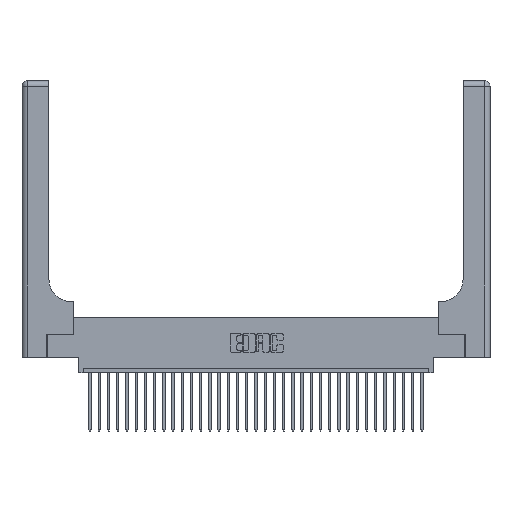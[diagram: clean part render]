
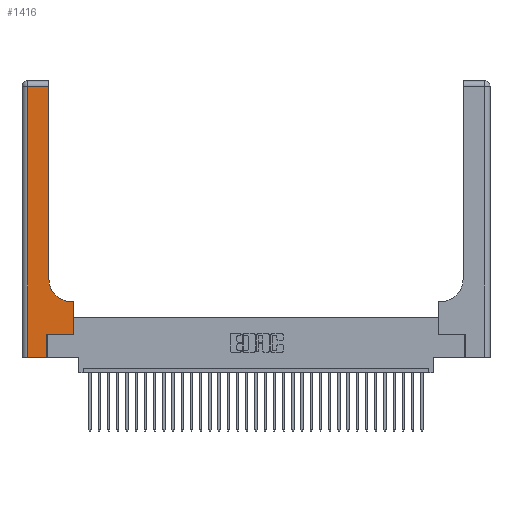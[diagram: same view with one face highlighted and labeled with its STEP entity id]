
A CAD part, top view. The second image highlights one B-rep face of the part: STEP entity #1416.
In plain terms, the highlighted planar face has unit normal (0, 0, 1).
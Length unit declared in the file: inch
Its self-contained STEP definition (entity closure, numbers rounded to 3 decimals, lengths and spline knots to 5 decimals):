
#181 = EDGE_CURVE ( 'NONE', #11528, #3983, #21302, .T. ) ;
#352 = DIRECTION ( 'NONE',  ( 0., 0., -1. ) ) ;
#624 = DIRECTION ( 'NONE',  ( -1., 0., 0. ) ) ;
#1255 = DIRECTION ( 'NONE',  ( 0., 1., 0. ) ) ;
#1416 = ADVANCED_FACE ( 'NONE', ( #32727 ), #31052, .F. ) ;
#1760 = LINE ( 'NONE', #19952, #2568 ) ;
#2340 = ORIENTED_EDGE ( 'NONE', *, *, #3587, .T. ) ;
#2445 = DIRECTION ( 'NONE',  ( -1., 0., 0. ) ) ;
#2512 = CARTESIAN_POINT ( 'NONE',  ( 0., 0., 0.37 ) ) ;
#2568 = VECTOR ( 'NONE', #9440, 39.37008 ) ;
#3167 = CARTESIAN_POINT ( 'NONE',  ( 0.06, 2.94, 0.37 ) ) ;
#3587 = EDGE_CURVE ( 'NONE', #3983, #24262, #4777, .T. ) ;
#3691 = ORIENTED_EDGE ( 'NONE', *, *, #11504, .T. ) ;
#3910 = DIRECTION ( 'NONE',  ( 1., 0., 0. ) ) ;
#3983 = VERTEX_POINT ( 'NONE', #8424 ) ;
#4261 = VERTEX_POINT ( 'NONE', #8640 ) ;
#4578 = DIRECTION ( 'NONE',  ( 1., 0., 0. ) ) ;
#4777 = LINE ( 'NONE', #16928, #6404 ) ;
#4928 = VECTOR ( 'NONE', #7871, 39.37008 ) ;
#5888 = VECTOR ( 'NONE', #25995, 39.37008 ) ;
#6015 = LINE ( 'NONE', #12961, #29697 ) ;
#6319 = CARTESIAN_POINT ( 'NONE',  ( 0.2915, 3., 0.37 ) ) ;
#6404 = VECTOR ( 'NONE', #4578, 39.37008 ) ;
#6488 = ORIENTED_EDGE ( 'NONE', *, *, #14481, .T. ) ;
#7114 = AXIS2_PLACEMENT_3D ( 'NONE', #13341, #16637, #18382 ) ;
#7279 = EDGE_LOOP ( 'NONE', ( #3691, #6488, #32698, #24462, #32759, #2340, #19197, #28678, #25270 ) ) ;
#7871 = DIRECTION ( 'NONE',  ( 1., 0., 0. ) ) ;
#8424 = CARTESIAN_POINT ( 'NONE',  ( 0.269, 0.25, 0.37 ) ) ;
#8640 = CARTESIAN_POINT ( 'NONE',  ( 0.2915, 2.94, 0.37 ) ) ;
#9211 = CARTESIAN_POINT ( 'NONE',  ( 0.269, 0., 0.37 ) ) ;
#9440 = DIRECTION ( 'NONE',  ( 0., -1., 0. ) ) ;
#9527 = VECTOR ( 'NONE', #624, 39.37008 ) ;
#10376 = VERTEX_POINT ( 'NONE', #3167 ) ;
#11504 = EDGE_CURVE ( 'NONE', #17576, #4261, #12606, .T. ) ;
#11528 = VERTEX_POINT ( 'NONE', #14206 ) ;
#12606 = LINE ( 'NONE', #6319, #15066 ) ;
#12929 = CARTESIAN_POINT ( 'NONE',  ( 0.2915, 0.85, 0.37 ) ) ;
#12961 = CARTESIAN_POINT ( 'NONE',  ( 0.2915, 0.6, 0.37 ) ) ;
#13341 = CARTESIAN_POINT ( 'NONE',  ( 0., 3., 0.37 ) ) ;
#14052 = LINE ( 'NONE', #29161, #9527 ) ;
#14206 = CARTESIAN_POINT ( 'NONE',  ( 0.269, 0., 0.37 ) ) ;
#14481 = EDGE_CURVE ( 'NONE', #4261, #10376, #14052, .T. ) ;
#14887 = EDGE_CURVE ( 'NONE', #10376, #19158, #1760, .T. ) ;
#15066 = VECTOR ( 'NONE', #27626, 39.37008 ) ;
#16047 = EDGE_CURVE ( 'NONE', #19158, #11528, #17182, .T. ) ;
#16442 = VERTEX_POINT ( 'NONE', #31165 ) ;
#16637 = DIRECTION ( 'NONE',  ( 0., 0., -1. ) ) ;
#16848 = VECTOR ( 'NONE', #1255, 39.37008 ) ;
#16928 = CARTESIAN_POINT ( 'NONE',  ( 0.269, 0.25, 0.37 ) ) ;
#17182 = LINE ( 'NONE', #2512, #4928 ) ;
#17576 = VERTEX_POINT ( 'NONE', #12929 ) ;
#18382 = DIRECTION ( 'NONE',  ( -1., 0., 0. ) ) ;
#18926 = EDGE_CURVE ( 'NONE', #16442, #25421, #6015, .T. ) ;
#18988 = EDGE_CURVE ( 'NONE', #25421, #17576, #23509, .T. ) ;
#19158 = VERTEX_POINT ( 'NONE', #27520 ) ;
#19197 = ORIENTED_EDGE ( 'NONE', *, *, #32466, .T. ) ;
#19952 = CARTESIAN_POINT ( 'NONE',  ( 0.06, 3., 0.37 ) ) ;
#20722 = CARTESIAN_POINT ( 'NONE',  ( 0.5415, 0.6, 0.37 ) ) ;
#21302 = LINE ( 'NONE', #9211, #16848 ) ;
#22152 = CARTESIAN_POINT ( 'NONE',  ( 0.5415, 0.85, 0.37 ) ) ;
#22614 = LINE ( 'NONE', #26102, #5888 ) ;
#23509 = CIRCLE ( 'NONE', #27486, 0.25 ) ;
#24262 = VERTEX_POINT ( 'NONE', #31128 ) ;
#24462 = ORIENTED_EDGE ( 'NONE', *, *, #16047, .T. ) ;
#25270 = ORIENTED_EDGE ( 'NONE', *, *, #18988, .T. ) ;
#25421 = VERTEX_POINT ( 'NONE', #20722 ) ;
#25995 = DIRECTION ( 'NONE',  ( 0., 1., 0. ) ) ;
#26102 = CARTESIAN_POINT ( 'NONE',  ( 0.5585, 0.25, 0.37 ) ) ;
#27486 = AXIS2_PLACEMENT_3D ( 'NONE', #22152, #352, #3910 ) ;
#27520 = CARTESIAN_POINT ( 'NONE',  ( 0.06, 0., 0.37 ) ) ;
#27626 = DIRECTION ( 'NONE',  ( 0., 1., 0. ) ) ;
#28678 = ORIENTED_EDGE ( 'NONE', *, *, #18926, .T. ) ;
#29161 = CARTESIAN_POINT ( 'NONE',  ( 0., 2.94, 0.37 ) ) ;
#29697 = VECTOR ( 'NONE', #2445, 39.37008 ) ;
#31052 = PLANE ( 'NONE',  #7114 ) ;
#31128 = CARTESIAN_POINT ( 'NONE',  ( 0.5585, 0.25, 0.37 ) ) ;
#31165 = CARTESIAN_POINT ( 'NONE',  ( 0.5585, 0.6, 0.37 ) ) ;
#32466 = EDGE_CURVE ( 'NONE', #24262, #16442, #22614, .T. ) ;
#32698 = ORIENTED_EDGE ( 'NONE', *, *, #14887, .T. ) ;
#32727 = FACE_OUTER_BOUND ( 'NONE', #7279, .T. ) ;
#32759 = ORIENTED_EDGE ( 'NONE', *, *, #181, .T. ) ;
